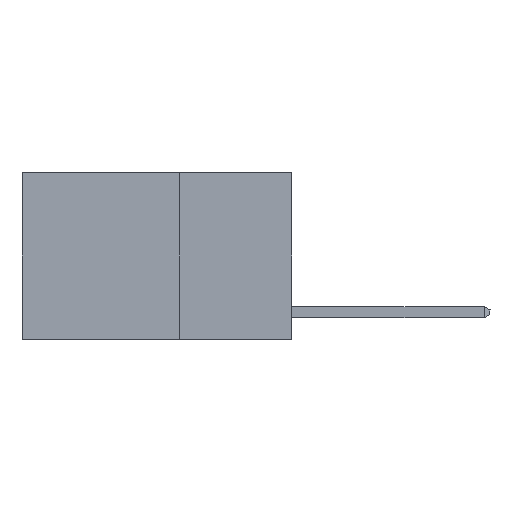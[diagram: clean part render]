
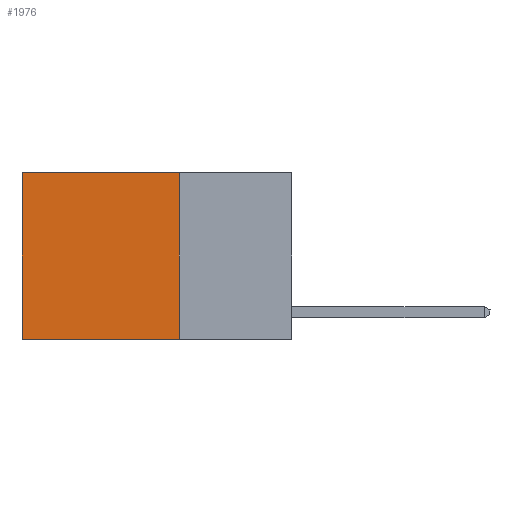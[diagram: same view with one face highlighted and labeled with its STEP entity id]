
A CAD part, left-side view. The second image highlights one B-rep face of the part: STEP entity #1976.
In plain terms, the highlighted planar face has unit normal (-1, 0, 0).
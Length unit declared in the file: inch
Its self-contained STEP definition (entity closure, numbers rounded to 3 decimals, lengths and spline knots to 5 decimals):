
#1086 = LINE ( 'NONE', #3689, #20434 ) ;
#1976 = ADVANCED_FACE ( 'NONE', ( #14634 ), #22106, .F. ) ;
#2770 = VERTEX_POINT ( 'NONE', #16676 ) ;
#2803 = CARTESIAN_POINT ( 'NONE',  ( 0.2625, 0.25, 0. ) ) ;
#2823 = CARTESIAN_POINT ( 'NONE',  ( 0.2625, 0.25, -0.37 ) ) ;
#3689 = CARTESIAN_POINT ( 'NONE',  ( 0.2625, 0.25, 0. ) ) ;
#3917 = CARTESIAN_POINT ( 'NONE',  ( 0.2625, 0.25, 0. ) ) ;
#6086 = VECTOR ( 'NONE', #23145, 39.37008 ) ;
#6563 = LINE ( 'NONE', #8879, #18534 ) ;
#8609 = AXIS2_PLACEMENT_3D ( 'NONE', #2803, #10310, #26809 ) ;
#8879 = CARTESIAN_POINT ( 'NONE',  ( 0.2625, 0.25, -0.37 ) ) ;
#8902 = CARTESIAN_POINT ( 'NONE',  ( 0.2625, 0.25, 0. ) ) ;
#10310 = DIRECTION ( 'NONE',  ( 1., 0., 0. ) ) ;
#11095 = LINE ( 'NONE', #19475, #14456 ) ;
#11656 = VERTEX_POINT ( 'NONE', #15767 ) ;
#12201 = EDGE_LOOP ( 'NONE', ( #23570, #23653, #19039, #19009 ) ) ;
#14456 = VECTOR ( 'NONE', #26654, 39.37008 ) ;
#14634 = FACE_OUTER_BOUND ( 'NONE', #12201, .T. ) ;
#15767 = CARTESIAN_POINT ( 'NONE',  ( 0.2625, 0.6, 0. ) ) ;
#15838 = DIRECTION ( 'NONE',  ( 0., 1., 0. ) ) ;
#15932 = EDGE_CURVE ( 'NONE', #27995, #2770, #6563, .T. ) ;
#16676 = CARTESIAN_POINT ( 'NONE',  ( 0.2625, 0.6, -0.37 ) ) ;
#17432 = VERTEX_POINT ( 'NONE', #8902 ) ;
#18534 = VECTOR ( 'NONE', #27760, 39.37008 ) ;
#19009 = ORIENTED_EDGE ( 'NONE', *, *, #23402, .T. ) ;
#19039 = ORIENTED_EDGE ( 'NONE', *, *, #26161, .F. ) ;
#19475 = CARTESIAN_POINT ( 'NONE',  ( 0.2625, 0.6, 0. ) ) ;
#20327 = LINE ( 'NONE', #3917, #6086 ) ;
#20434 = VECTOR ( 'NONE', #15838, 39.37008 ) ;
#22106 = PLANE ( 'NONE',  #8609 ) ;
#23145 = DIRECTION ( 'NONE',  ( 0., 0., -1. ) ) ;
#23402 = EDGE_CURVE ( 'NONE', #17432, #11656, #1086, .T. ) ;
#23570 = ORIENTED_EDGE ( 'NONE', *, *, #29403, .T. ) ;
#23653 = ORIENTED_EDGE ( 'NONE', *, *, #15932, .F. ) ;
#26161 = EDGE_CURVE ( 'NONE', #17432, #27995, #20327, .T. ) ;
#26654 = DIRECTION ( 'NONE',  ( 0., 0., -1. ) ) ;
#26809 = DIRECTION ( 'NONE',  ( 0., 0., -1. ) ) ;
#27760 = DIRECTION ( 'NONE',  ( 0., 1., 0. ) ) ;
#27995 = VERTEX_POINT ( 'NONE', #2823 ) ;
#29403 = EDGE_CURVE ( 'NONE', #11656, #2770, #11095, .T. ) ;
